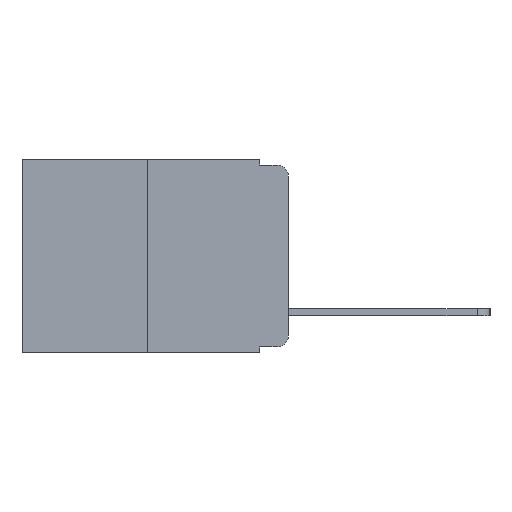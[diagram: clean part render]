
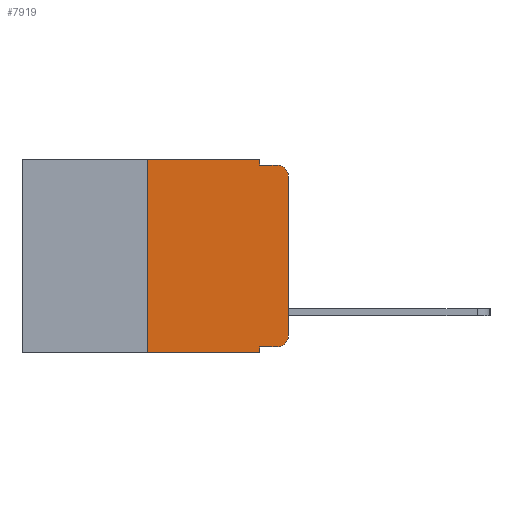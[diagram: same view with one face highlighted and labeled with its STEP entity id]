
A CAD part, left-side view. The second image highlights one B-rep face of the part: STEP entity #7919.
In plain terms, the highlighted planar face has unit normal (-1, 0, 0).
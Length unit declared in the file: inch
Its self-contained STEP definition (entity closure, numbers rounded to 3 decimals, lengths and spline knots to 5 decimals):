
#210 = VECTOR ( 'NONE', #512, 39.37008 ) ;
#273 = CARTESIAN_POINT ( 'NONE',  ( 0., 0.25, -0.343 ) ) ;
#319 = AXIS2_PLACEMENT_3D ( 'NONE', #5148, #9775, #5188 ) ;
#416 = ORIENTED_EDGE ( 'NONE', *, *, #1839, .F. ) ;
#509 = EDGE_CURVE ( 'NONE', #6609, #9373, #9567, .T. ) ;
#512 = DIRECTION ( 'NONE',  ( 0., 0., -1. ) ) ;
#615 = VECTOR ( 'NONE', #5458, 39.37008 ) ;
#755 = ORIENTED_EDGE ( 'NONE', *, *, #1838, .T. ) ;
#956 = VECTOR ( 'NONE', #9006, 39.37008 ) ;
#1010 = CARTESIAN_POINT ( 'NONE',  ( 0., 0.051, -0.343 ) ) ;
#1117 = VERTEX_POINT ( 'NONE', #1010 ) ;
#1251 = EDGE_CURVE ( 'NONE', #2194, #1117, #4091, .T. ) ;
#1823 = EDGE_CURVE ( 'NONE', #7644, #9969, #6754, .T. ) ;
#1838 = EDGE_CURVE ( 'NONE', #9969, #3872, #6514, .T. ) ;
#1839 = EDGE_CURVE ( 'NONE', #9606, #3872, #6264, .T. ) ;
#1861 = EDGE_CURVE ( 'NONE', #9373, #9606, #3534, .T. ) ;
#1879 = EDGE_CURVE ( 'NONE', #2194, #6609, #7824, .T. ) ;
#1884 = EDGE_CURVE ( 'NONE', #6926, #1117, #6005, .T. ) ;
#1917 = EDGE_CURVE ( 'NONE', #6926, #3138, #9530, .T. ) ;
#1918 = EDGE_CURVE ( 'NONE', #3138, #7644, #2809, .T. ) ;
#2088 = DIRECTION ( 'NONE',  ( -1., 0., 0. ) ) ;
#2194 = VERTEX_POINT ( 'NONE', #273 ) ;
#2663 = CARTESIAN_POINT ( 'NONE',  ( 0., 0.051, -0.01 ) ) ;
#2809 = CIRCLE ( 'NONE', #9798, 0.02 ) ;
#2868 = VECTOR ( 'NONE', #4298, 39.37008 ) ;
#3138 = VERTEX_POINT ( 'NONE', #11128 ) ;
#3158 = CARTESIAN_POINT ( 'NONE',  ( 0., 0.25, 0. ) ) ;
#3179 = VECTOR ( 'NONE', #11343, 39.37008 ) ;
#3534 = LINE ( 'NONE', #9314, #615 ) ;
#3652 = ORIENTED_EDGE ( 'NONE', *, *, #1918, .T. ) ;
#3872 = VERTEX_POINT ( 'NONE', #7755 ) ;
#4091 = LINE ( 'NONE', #4499, #9440 ) ;
#4204 = CARTESIAN_POINT ( 'NONE',  ( 0., 0., 0. ) ) ;
#4267 = PLANE ( 'NONE',  #319 ) ;
#4275 = ORIENTED_EDGE ( 'NONE', *, *, #1861, .F. ) ;
#4298 = DIRECTION ( 'NONE',  ( 0., -1., 0. ) ) ;
#4336 = EDGE_LOOP ( 'NONE', ( #4595, #755, #416, #4275, #4817, #7075, #6376, #5261, #4684, #3652 ) ) ;
#4499 = CARTESIAN_POINT ( 'NONE',  ( 0., 0.473, -0.343 ) ) ;
#4555 = VECTOR ( 'NONE', #6072, 39.37008 ) ;
#4595 = ORIENTED_EDGE ( 'NONE', *, *, #1823, .T. ) ;
#4684 = ORIENTED_EDGE ( 'NONE', *, *, #1917, .T. ) ;
#4817 = ORIENTED_EDGE ( 'NONE', *, *, #509, .F. ) ;
#5148 = CARTESIAN_POINT ( 'NONE',  ( 0., 0.473, 0. ) ) ;
#5188 = DIRECTION ( 'NONE',  ( 0., 0., -1. ) ) ;
#5261 = ORIENTED_EDGE ( 'NONE', *, *, #1884, .F. ) ;
#5458 = DIRECTION ( 'NONE',  ( 0., 0., -1. ) ) ;
#5746 = VECTOR ( 'NONE', #7575, 39.37008 ) ;
#6005 = LINE ( 'NONE', #9517, #210 ) ;
#6072 = DIRECTION ( 'NONE',  ( 0., 0., 1. ) ) ;
#6252 = CARTESIAN_POINT ( 'NONE',  ( 0., 0.051, 0. ) ) ;
#6264 = LINE ( 'NONE', #7114, #956 ) ;
#6376 = ORIENTED_EDGE ( 'NONE', *, *, #1251, .T. ) ;
#6514 = CIRCLE ( 'NONE', #9849, 0.02 ) ;
#6609 = VERTEX_POINT ( 'NONE', #3158 ) ;
#6754 = LINE ( 'NONE', #4204, #4555 ) ;
#6866 = CARTESIAN_POINT ( 'NONE',  ( 0., 0.473, 0. ) ) ;
#6871 = DIRECTION ( 'NONE',  ( 0., 0., -1. ) ) ;
#6926 = VERTEX_POINT ( 'NONE', #9234 ) ;
#7075 = ORIENTED_EDGE ( 'NONE', *, *, #1879, .F. ) ;
#7114 = CARTESIAN_POINT ( 'NONE',  ( 0., 0.051, -0.01 ) ) ;
#7575 = DIRECTION ( 'NONE',  ( 0., 0., 1. ) ) ;
#7644 = VERTEX_POINT ( 'NONE', #10258 ) ;
#7718 = DIRECTION ( 'NONE',  ( -1., 0., 0. ) ) ;
#7755 = CARTESIAN_POINT ( 'NONE',  ( 0., 0.02, -0.01 ) ) ;
#7824 = LINE ( 'NONE', #9226, #5746 ) ;
#7919 = ADVANCED_FACE ( 'NONE', ( #10995 ), #4267, .F. ) ;
#8324 = CARTESIAN_POINT ( 'NONE',  ( 0., 0., -0.03 ) ) ;
#8369 = CARTESIAN_POINT ( 'NONE',  ( 0., 0.02, -0.03 ) ) ;
#8536 = CARTESIAN_POINT ( 'NONE',  ( 0., 0.051, -0.333 ) ) ;
#9006 = DIRECTION ( 'NONE',  ( 0., -1., 0. ) ) ;
#9226 = CARTESIAN_POINT ( 'NONE',  ( 0., 0.25, 0. ) ) ;
#9234 = CARTESIAN_POINT ( 'NONE',  ( 0., 0.051, -0.333 ) ) ;
#9314 = CARTESIAN_POINT ( 'NONE',  ( 0., 0.051, 0. ) ) ;
#9373 = VERTEX_POINT ( 'NONE', #6252 ) ;
#9415 = DIRECTION ( 'NONE',  ( 0., -1., 0. ) ) ;
#9435 = CARTESIAN_POINT ( 'NONE',  ( 0., 0.02, -0.313 ) ) ;
#9440 = VECTOR ( 'NONE', #9415, 39.37008 ) ;
#9517 = CARTESIAN_POINT ( 'NONE',  ( 0., 0.051, 0. ) ) ;
#9530 = LINE ( 'NONE', #8536, #3179 ) ;
#9567 = LINE ( 'NONE', #6866, #2868 ) ;
#9606 = VERTEX_POINT ( 'NONE', #2663 ) ;
#9775 = DIRECTION ( 'NONE',  ( 1., 0., 0. ) ) ;
#9798 = AXIS2_PLACEMENT_3D ( 'NONE', #9435, #7718, #6871 ) ;
#9849 = AXIS2_PLACEMENT_3D ( 'NONE', #8369, #2088, #11254 ) ;
#9969 = VERTEX_POINT ( 'NONE', #8324 ) ;
#10258 = CARTESIAN_POINT ( 'NONE',  ( 0., 0., -0.313 ) ) ;
#10995 = FACE_OUTER_BOUND ( 'NONE', #4336, .T. ) ;
#11128 = CARTESIAN_POINT ( 'NONE',  ( 0., 0.02, -0.333 ) ) ;
#11254 = DIRECTION ( 'NONE',  ( 0., 0., -1. ) ) ;
#11343 = DIRECTION ( 'NONE',  ( 0., -1., 0. ) ) ;
